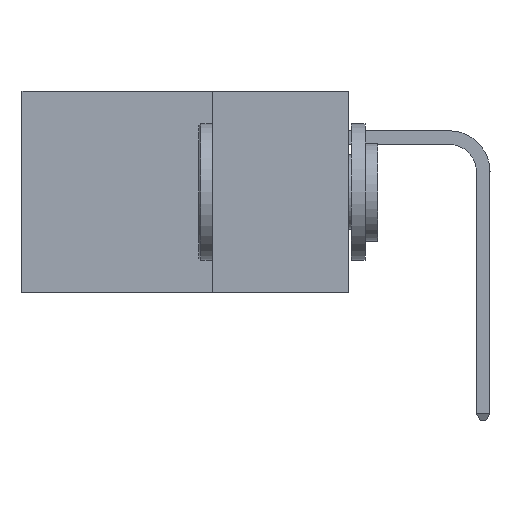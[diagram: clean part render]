
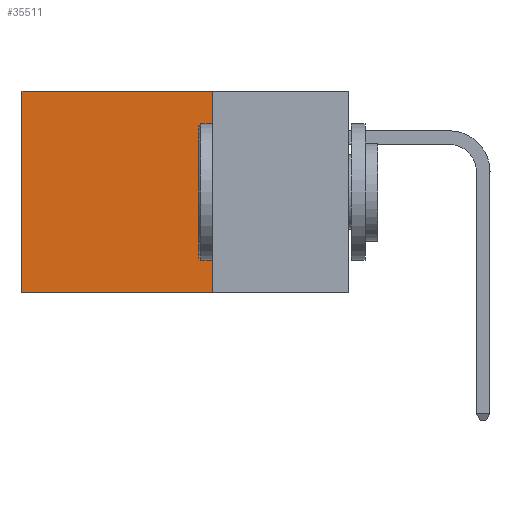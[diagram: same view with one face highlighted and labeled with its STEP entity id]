
A CAD part, left-side view. The second image highlights one B-rep face of the part: STEP entity #35511.
In plain terms, the highlighted planar face has unit normal (-1, 0, 0).
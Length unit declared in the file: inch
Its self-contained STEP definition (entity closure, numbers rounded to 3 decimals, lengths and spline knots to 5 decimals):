
#123 = DIRECTION ( 'NONE',  ( 0., 0., -1. ) ) ;
#255 = VECTOR ( 'NONE', #18271, 39.37008 ) ;
#444 = VERTEX_POINT ( 'NONE', #20886 ) ;
#2340 = FACE_OUTER_BOUND ( 'NONE', #36370, .T. ) ;
#2461 = CARTESIAN_POINT ( 'NONE',  ( 0.2875, 0.25, 0. ) ) ;
#3658 = CARTESIAN_POINT ( 'NONE',  ( 0.2875, 0.25, 0. ) ) ;
#5772 = VERTEX_POINT ( 'NONE', #3658 ) ;
#5904 = LINE ( 'NONE', #27650, #27417 ) ;
#5929 = CARTESIAN_POINT ( 'NONE',  ( 0.2875, 0.6, 0. ) ) ;
#6191 = EDGE_CURVE ( 'NONE', #5772, #15456, #14067, .T. ) ;
#8913 = CARTESIAN_POINT ( 'NONE',  ( 0.2875, 0.25, 0. ) ) ;
#9558 = CARTESIAN_POINT ( 'NONE',  ( 0.2875, 0.25, -0.37 ) ) ;
#10127 = DIRECTION ( 'NONE',  ( 0., 1., 0. ) ) ;
#11045 = EDGE_CURVE ( 'NONE', #22866, #444, #30607, .T. ) ;
#11371 = DIRECTION ( 'NONE',  ( 0., 0., -1. ) ) ;
#14067 = LINE ( 'NONE', #2461, #19070 ) ;
#15222 = CARTESIAN_POINT ( 'NONE',  ( 0.2875, 0.25, 0. ) ) ;
#15456 = VERTEX_POINT ( 'NONE', #9558 ) ;
#15878 = ORIENTED_EDGE ( 'NONE', *, *, #27692, .F. ) ;
#17342 = ORIENTED_EDGE ( 'NONE', *, *, #11045, .T. ) ;
#17752 = DIRECTION ( 'NONE',  ( 1., 0., 0. ) ) ;
#18271 = DIRECTION ( 'NONE',  ( 0., 1., 0. ) ) ;
#18680 = LINE ( 'NONE', #15222, #255 ) ;
#19070 = VECTOR ( 'NONE', #11371, 39.37008 ) ;
#20886 = CARTESIAN_POINT ( 'NONE',  ( 0.2875, 0.6, -0.37 ) ) ;
#21441 = EDGE_CURVE ( 'NONE', #5772, #22866, #18680, .T. ) ;
#22866 = VERTEX_POINT ( 'NONE', #27637 ) ;
#23768 = VECTOR ( 'NONE', #26407, 39.37008 ) ;
#26407 = DIRECTION ( 'NONE',  ( 0., 0., -1. ) ) ;
#27389 = AXIS2_PLACEMENT_3D ( 'NONE', #8913, #17752, #123 ) ;
#27417 = VECTOR ( 'NONE', #10127, 39.37008 ) ;
#27637 = CARTESIAN_POINT ( 'NONE',  ( 0.2875, 0.6, 0. ) ) ;
#27650 = CARTESIAN_POINT ( 'NONE',  ( 0.2875, 0.25, -0.37 ) ) ;
#27692 = EDGE_CURVE ( 'NONE', #15456, #444, #5904, .T. ) ;
#30607 = LINE ( 'NONE', #5929, #23768 ) ;
#33832 = ORIENTED_EDGE ( 'NONE', *, *, #6191, .F. ) ;
#35216 = PLANE ( 'NONE',  #27389 ) ;
#35511 = ADVANCED_FACE ( 'NONE', ( #2340 ), #35216, .F. ) ;
#36370 = EDGE_LOOP ( 'NONE', ( #17342, #15878, #33832, #37161 ) ) ;
#37161 = ORIENTED_EDGE ( 'NONE', *, *, #21441, .T. ) ;
